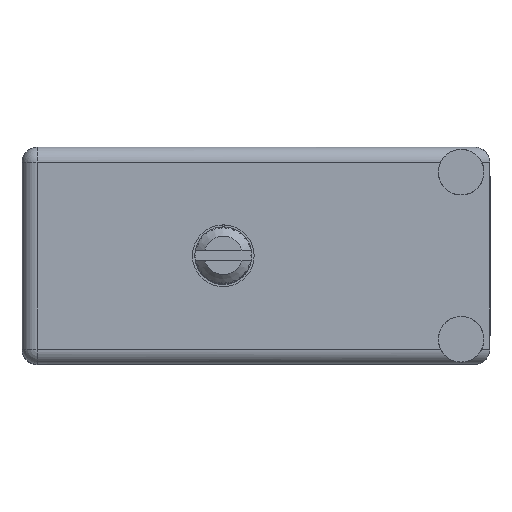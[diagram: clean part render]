
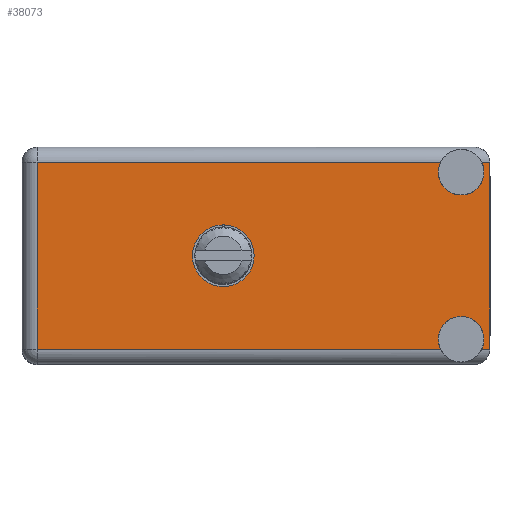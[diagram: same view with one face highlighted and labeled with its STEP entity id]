
A CAD part, top view. The second image highlights one B-rep face of the part: STEP entity #38073.
In plain terms, the highlighted face is planar.
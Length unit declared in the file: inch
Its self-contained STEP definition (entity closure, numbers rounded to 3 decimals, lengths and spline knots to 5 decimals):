
#484 = DIRECTION ( 'NONE',  ( 0., 1., 0. ) ) ;
#7500 = CARTESIAN_POINT ( 'NONE',  ( -0.6125, 0.806, -0.3075 ) ) ;
#8347 = CARTESIAN_POINT ( 'NONE',  ( 0., 0.806, 0. ) ) ;
#9399 = EDGE_CURVE ( 'NONE', #179809, #151341, #118228, .T. ) ;
#12785 = ORIENTED_EDGE ( 'NONE', *, *, #44094, .T. ) ;
#19096 = VECTOR ( 'NONE', #66769, 39.37008 ) ;
#20528 = CARTESIAN_POINT ( 'NONE',  ( -0.6625, 0.806, -0.3075 ) ) ;
#21703 = EDGE_CURVE ( 'NONE', #111899, #115013, #27343, .T. ) ;
#23013 = VECTOR ( 'NONE', #85638, 39.37008 ) ;
#23718 = LINE ( 'NONE', #20528, #66955 ) ;
#23775 = DIRECTION ( 'NONE',  ( 0., 0., 1. ) ) ;
#23972 = DIRECTION ( 'NONE',  ( 0., 1., 0. ) ) ;
#26412 = CARTESIAN_POINT ( 'NONE',  ( 0.71491, 0.806, -0.3075 ) ) ;
#27343 = CIRCLE ( 'NONE', #114149, 0.1015 ) ;
#33828 = CIRCLE ( 'NONE', #198725, 0.075 ) ;
#35419 = CARTESIAN_POINT ( 'NONE',  ( 0., 0.806, -0.1015 ) ) ;
#38073 = ADVANCED_FACE ( 'NONE', ( #101102, #125379 ), #87964, .T. ) ;
#40316 = CIRCLE ( 'NONE', #144067, 0.075 ) ;
#42013 = CARTESIAN_POINT ( 'NONE',  ( 0., 0.806, 0.1015 ) ) ;
#42323 = CARTESIAN_POINT ( 'NONE',  ( 0.8765, 0.806, 0.3075 ) ) ;
#44094 = EDGE_CURVE ( 'NONE', #151341, #63613, #76034, .T. ) ;
#45765 = CARTESIAN_POINT ( 'NONE',  ( 0.85009, 0.806, 0.3075 ) ) ;
#47043 = VERTEX_POINT ( 'NONE', #42323 ) ;
#53734 = VERTEX_POINT ( 'NONE', #26412 ) ;
#54956 = CIRCLE ( 'NONE', #172387, 0.075 ) ;
#56412 = DIRECTION ( 'NONE',  ( -1., 0., 0. ) ) ;
#62027 = CARTESIAN_POINT ( 'NONE',  ( -0.6125, 0.806, -0.3575 ) ) ;
#63613 = VERTEX_POINT ( 'NONE', #73089 ) ;
#63717 = ORIENTED_EDGE ( 'NONE', *, *, #92734, .F. ) ;
#64923 = DIRECTION ( 'NONE',  ( -1., 0., 0. ) ) ;
#66769 = DIRECTION ( 'NONE',  ( -1., 0., 0. ) ) ;
#66955 = VECTOR ( 'NONE', #64923, 39.37008 ) ;
#73089 = CARTESIAN_POINT ( 'NONE',  ( 0.71491, 0.806, 0.3075 ) ) ;
#73575 = EDGE_CURVE ( 'NONE', #115013, #111899, #164172, .T. ) ;
#76034 = LINE ( 'NONE', #79680, #92834 ) ;
#77197 = AXIS2_PLACEMENT_3D ( 'NONE', #8347, #133531, #101803 ) ;
#79680 = CARTESIAN_POINT ( 'NONE',  ( 0.8765, 0.806, 0.3075 ) ) ;
#85638 = DIRECTION ( 'NONE',  ( 0., 0., 1. ) ) ;
#87964 = PLANE ( 'NONE',  #140337 ) ;
#88098 = VERTEX_POINT ( 'NONE', #100395 ) ;
#91294 = ORIENTED_EDGE ( 'NONE', *, *, #148954, .F. ) ;
#92734 = EDGE_CURVE ( 'NONE', #96039, #88098, #33828, .T. ) ;
#92834 = VECTOR ( 'NONE', #93847, 39.37008 ) ;
#93847 = DIRECTION ( 'NONE',  ( 1., 0., 0. ) ) ;
#94935 = ORIENTED_EDGE ( 'NONE', *, *, #9399, .T. ) ;
#96039 = VERTEX_POINT ( 'NONE', #45765 ) ;
#100395 = CARTESIAN_POINT ( 'NONE',  ( 0.7825, 0.806, 0.2 ) ) ;
#101102 = FACE_BOUND ( 'NONE', #104909, .T. ) ;
#101297 = CARTESIAN_POINT ( 'NONE',  ( 0.7825, 0.806, -0.275 ) ) ;
#101472 = DIRECTION ( 'NONE',  ( 0., 1., 0. ) ) ;
#101575 = DIRECTION ( 'NONE',  ( 1., 0., 0. ) ) ;
#101803 = DIRECTION ( 'NONE',  ( 0., 0., 1. ) ) ;
#104909 = EDGE_LOOP ( 'NONE', ( #162994, #108068 ) ) ;
#105469 = EDGE_CURVE ( 'NONE', #107875, #161198, #54956, .T. ) ;
#107875 = VERTEX_POINT ( 'NONE', #181845 ) ;
#108068 = ORIENTED_EDGE ( 'NONE', *, *, #21703, .F. ) ;
#111899 = VERTEX_POINT ( 'NONE', #35419 ) ;
#112281 = EDGE_CURVE ( 'NONE', #189162, #161198, #192444, .T. ) ;
#113397 = VECTOR ( 'NONE', #137475, 39.37008 ) ;
#114149 = AXIS2_PLACEMENT_3D ( 'NONE', #155235, #484, #139795 ) ;
#115013 = VERTEX_POINT ( 'NONE', #42013 ) ;
#116174 = CARTESIAN_POINT ( 'NONE',  ( 0.7825, 0.806, -0.275 ) ) ;
#118228 = LINE ( 'NONE', #62027, #113397 ) ;
#118358 = CARTESIAN_POINT ( 'NONE',  ( -0.6625, 0.806, -0.3575 ) ) ;
#119367 = ORIENTED_EDGE ( 'NONE', *, *, #112281, .T. ) ;
#125379 = FACE_OUTER_BOUND ( 'NONE', #166233, .T. ) ;
#131442 = DIRECTION ( 'NONE',  ( 0., 1., 0. ) ) ;
#131626 = DIRECTION ( 'NONE',  ( 0., 0., 1. ) ) ;
#133531 = DIRECTION ( 'NONE',  ( 0., 1., 0. ) ) ;
#137475 = DIRECTION ( 'NONE',  ( 0., 0., 1. ) ) ;
#138738 = ORIENTED_EDGE ( 'NONE', *, *, #148599, .T. ) ;
#139795 = DIRECTION ( 'NONE',  ( 0., 0., 1. ) ) ;
#140337 = AXIS2_PLACEMENT_3D ( 'NONE', #118358, #101472, #56412 ) ;
#143250 = LINE ( 'NONE', #192462, #171924 ) ;
#144067 = AXIS2_PLACEMENT_3D ( 'NONE', #116174, #23972, #131626 ) ;
#145631 = ORIENTED_EDGE ( 'NONE', *, *, #182741, .F. ) ;
#146372 = AXIS2_PLACEMENT_3D ( 'NONE', #177090, #131442, #23775 ) ;
#148599 = EDGE_CURVE ( 'NONE', #53734, #179809, #23718, .T. ) ;
#148954 = EDGE_CURVE ( 'NONE', #53734, #107875, #40316, .T. ) ;
#151341 = VERTEX_POINT ( 'NONE', #177604 ) ;
#152958 = LINE ( 'NONE', #163031, #23013 ) ;
#155235 = CARTESIAN_POINT ( 'NONE',  ( 0., 0.806, 0. ) ) ;
#155780 = CARTESIAN_POINT ( 'NONE',  ( 0.7825, 0.806, 0.275 ) ) ;
#159106 = CIRCLE ( 'NONE', #146372, 0.075 ) ;
#161198 = VERTEX_POINT ( 'NONE', #165854 ) ;
#162994 = ORIENTED_EDGE ( 'NONE', *, *, #73575, .F. ) ;
#163031 = CARTESIAN_POINT ( 'NONE',  ( 0.8765, 0.806, 0.3575 ) ) ;
#163202 = DIRECTION ( 'NONE',  ( 0., 0., 1. ) ) ;
#163638 = ORIENTED_EDGE ( 'NONE', *, *, #175366, .F. ) ;
#164172 = CIRCLE ( 'NONE', #77197, 0.1015 ) ;
#165854 = CARTESIAN_POINT ( 'NONE',  ( 0.85009, 0.806, -0.3075 ) ) ;
#166233 = EDGE_LOOP ( 'NONE', ( #12785, #163638, #63717, #195473, #145631, #119367, #169759, #91294, #138738, #94935 ) ) ;
#169759 = ORIENTED_EDGE ( 'NONE', *, *, #105469, .F. ) ;
#170910 = EDGE_CURVE ( 'NONE', #96039, #47043, #143250, .T. ) ;
#171841 = DIRECTION ( 'NONE',  ( 0., 0., 1. ) ) ;
#171924 = VECTOR ( 'NONE', #101575, 39.37008 ) ;
#172387 = AXIS2_PLACEMENT_3D ( 'NONE', #101297, #179961, #163202 ) ;
#175366 = EDGE_CURVE ( 'NONE', #88098, #63613, #159106, .T. ) ;
#177090 = CARTESIAN_POINT ( 'NONE',  ( 0.7825, 0.806, 0.275 ) ) ;
#177604 = CARTESIAN_POINT ( 'NONE',  ( -0.6125, 0.806, 0.3075 ) ) ;
#179809 = VERTEX_POINT ( 'NONE', #7500 ) ;
#179961 = DIRECTION ( 'NONE',  ( 0., 1., 0. ) ) ;
#181845 = CARTESIAN_POINT ( 'NONE',  ( 0.7825, 0.806, -0.2 ) ) ;
#182569 = DIRECTION ( 'NONE',  ( 0., 1., 0. ) ) ;
#182741 = EDGE_CURVE ( 'NONE', #189162, #47043, #152958, .T. ) ;
#186167 = CARTESIAN_POINT ( 'NONE',  ( 0.8765, 0.806, -0.3075 ) ) ;
#189162 = VERTEX_POINT ( 'NONE', #186167 ) ;
#191199 = CARTESIAN_POINT ( 'NONE',  ( -0.6625, 0.806, -0.3075 ) ) ;
#192444 = LINE ( 'NONE', #191199, #19096 ) ;
#192462 = CARTESIAN_POINT ( 'NONE',  ( 0.8765, 0.806, 0.3075 ) ) ;
#195473 = ORIENTED_EDGE ( 'NONE', *, *, #170910, .T. ) ;
#198725 = AXIS2_PLACEMENT_3D ( 'NONE', #155780, #182569, #171841 ) ;
